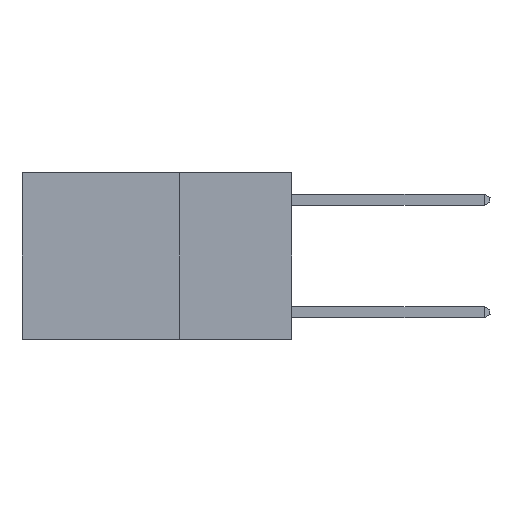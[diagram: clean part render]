
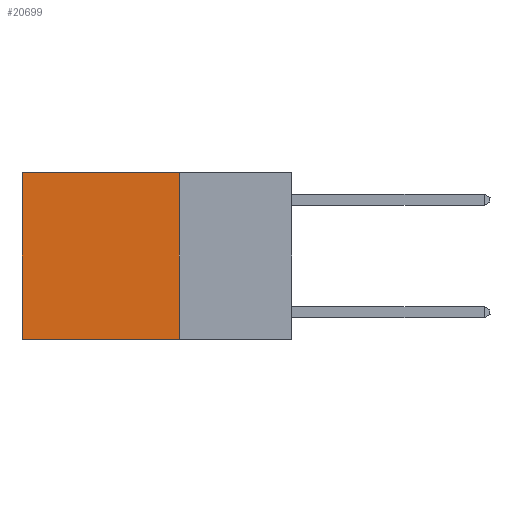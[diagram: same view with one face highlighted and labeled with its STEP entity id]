
A CAD part, left-side view. The second image highlights one B-rep face of the part: STEP entity #20699.
In plain terms, the highlighted planar face has unit normal (-1, 0, 0).
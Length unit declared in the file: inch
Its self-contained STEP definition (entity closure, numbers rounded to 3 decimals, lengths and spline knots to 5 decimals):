
#1035 = DIRECTION ( 'NONE',  ( 1., 0., 0. ) ) ;
#1456 = DIRECTION ( 'NONE',  ( 0., 0., -1. ) ) ;
#1516 = VERTEX_POINT ( 'NONE', #6463 ) ;
#2877 = FACE_OUTER_BOUND ( 'NONE', #6125, .T. ) ;
#3262 = VECTOR ( 'NONE', #13944, 39.37008 ) ;
#3780 = VERTEX_POINT ( 'NONE', #11949 ) ;
#4527 = CARTESIAN_POINT ( 'NONE',  ( 0.2625, 0.6, -0.37 ) ) ;
#4659 = ORIENTED_EDGE ( 'NONE', *, *, #9175, .T. ) ;
#5744 = DIRECTION ( 'NONE',  ( 0., 0., -1. ) ) ;
#6125 = EDGE_LOOP ( 'NONE', ( #4659, #9839, #15468, #13726 ) ) ;
#6129 = CARTESIAN_POINT ( 'NONE',  ( 0.2625, 0.25, 0. ) ) ;
#6463 = CARTESIAN_POINT ( 'NONE',  ( 0.2625, 0.25, -0.37 ) ) ;
#6854 = DIRECTION ( 'NONE',  ( 0., 1., 0. ) ) ;
#6926 = CARTESIAN_POINT ( 'NONE',  ( 0.2625, 0.6, 0. ) ) ;
#7144 = LINE ( 'NONE', #20395, #7633 ) ;
#7470 = EDGE_CURVE ( 'NONE', #3780, #12892, #10056, .T. ) ;
#7633 = VECTOR ( 'NONE', #5744, 39.37008 ) ;
#9175 = EDGE_CURVE ( 'NONE', #12892, #14447, #7144, .T. ) ;
#9194 = CARTESIAN_POINT ( 'NONE',  ( 0.2625, 0.25, 0. ) ) ;
#9839 = ORIENTED_EDGE ( 'NONE', *, *, #15340, .F. ) ;
#10056 = LINE ( 'NONE', #11881, #13744 ) ;
#10842 = LINE ( 'NONE', #12130, #3262 ) ;
#11881 = CARTESIAN_POINT ( 'NONE',  ( 0.2625, 0.25, 0. ) ) ;
#11949 = CARTESIAN_POINT ( 'NONE',  ( 0.2625, 0.25, 0. ) ) ;
#12130 = CARTESIAN_POINT ( 'NONE',  ( 0.2625, 0.25, -0.37 ) ) ;
#12823 = PLANE ( 'NONE',  #12935 ) ;
#12892 = VERTEX_POINT ( 'NONE', #6926 ) ;
#12935 = AXIS2_PLACEMENT_3D ( 'NONE', #9194, #1035, #1456 ) ;
#12992 = DIRECTION ( 'NONE',  ( 0., 0., -1. ) ) ;
#13726 = ORIENTED_EDGE ( 'NONE', *, *, #7470, .T. ) ;
#13744 = VECTOR ( 'NONE', #6854, 39.37008 ) ;
#13944 = DIRECTION ( 'NONE',  ( 0., 1., 0. ) ) ;
#14447 = VERTEX_POINT ( 'NONE', #4527 ) ;
#14703 = LINE ( 'NONE', #6129, #16703 ) ;
#15340 = EDGE_CURVE ( 'NONE', #1516, #14447, #10842, .T. ) ;
#15468 = ORIENTED_EDGE ( 'NONE', *, *, #16329, .F. ) ;
#16329 = EDGE_CURVE ( 'NONE', #3780, #1516, #14703, .T. ) ;
#16703 = VECTOR ( 'NONE', #12992, 39.37008 ) ;
#20395 = CARTESIAN_POINT ( 'NONE',  ( 0.2625, 0.6, 0. ) ) ;
#20699 = ADVANCED_FACE ( 'NONE', ( #2877 ), #12823, .F. ) ;
